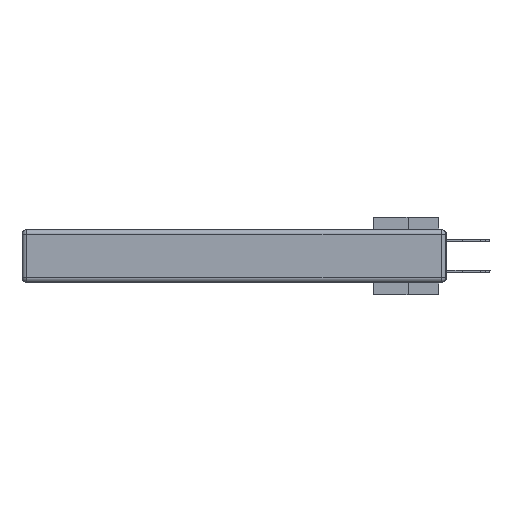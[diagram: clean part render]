
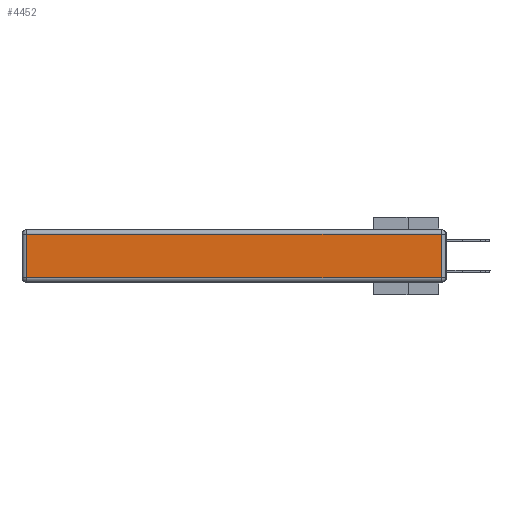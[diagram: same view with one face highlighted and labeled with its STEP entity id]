
A CAD part, left-side view. The second image highlights one B-rep face of the part: STEP entity #4452.
In plain terms, the highlighted planar face has unit normal (-1, 0, 0).
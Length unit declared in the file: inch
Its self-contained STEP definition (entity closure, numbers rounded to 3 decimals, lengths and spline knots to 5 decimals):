
#385 = VERTEX_POINT ( 'NONE', #31252 ) ;
#1004 = EDGE_CURVE ( 'NONE', #385, #21930, #6210, .T. ) ;
#1179 = CARTESIAN_POINT ( 'NONE',  ( 0., 2.72, -0.343 ) ) ;
#1452 = CARTESIAN_POINT ( 'NONE',  ( 0., 0.03, -0.313 ) ) ;
#2350 = EDGE_LOOP ( 'NONE', ( #24834, #15206, #16916, #13776 ) ) ;
#3061 = VECTOR ( 'NONE', #31556, 39.37008 ) ;
#4452 = ADVANCED_FACE ( 'NONE', ( #31015 ), #16796, .T. ) ;
#5399 = EDGE_CURVE ( 'NONE', #21930, #14208, #33611, .T. ) ;
#5431 = DIRECTION ( 'NONE',  ( -1., 0., 0. ) ) ;
#5681 = CARTESIAN_POINT ( 'NONE',  ( 0., 0.03, -0.343 ) ) ;
#6210 = LINE ( 'NONE', #35087, #19211 ) ;
#7542 = LINE ( 'NONE', #1179, #27296 ) ;
#12952 = AXIS2_PLACEMENT_3D ( 'NONE', #22569, #5431, #36917 ) ;
#13776 = ORIENTED_EDGE ( 'NONE', *, *, #34782, .T. ) ;
#14208 = VERTEX_POINT ( 'NONE', #25687 ) ;
#15206 = ORIENTED_EDGE ( 'NONE', *, *, #5399, .T. ) ;
#16582 = DIRECTION ( 'NONE',  ( 0., 0., 1. ) ) ;
#16702 = EDGE_CURVE ( 'NONE', #14208, #31904, #22338, .T. ) ;
#16796 = PLANE ( 'NONE',  #12952 ) ;
#16916 = ORIENTED_EDGE ( 'NONE', *, *, #16702, .T. ) ;
#19211 = VECTOR ( 'NONE', #29871, 39.37008 ) ;
#21930 = VERTEX_POINT ( 'NONE', #1452 ) ;
#22338 = LINE ( 'NONE', #26167, #3061 ) ;
#22569 = CARTESIAN_POINT ( 'NONE',  ( 0., 0., -0.343 ) ) ;
#24834 = ORIENTED_EDGE ( 'NONE', *, *, #1004, .T. ) ;
#25687 = CARTESIAN_POINT ( 'NONE',  ( 0., 0.03, -0.03 ) ) ;
#26167 = CARTESIAN_POINT ( 'NONE',  ( 0., 2.75, -0.03 ) ) ;
#26557 = CARTESIAN_POINT ( 'NONE',  ( 0., 2.72, -0.03 ) ) ;
#27296 = VECTOR ( 'NONE', #33094, 39.37008 ) ;
#27367 = VECTOR ( 'NONE', #16582, 39.37008 ) ;
#29871 = DIRECTION ( 'NONE',  ( 0., -1., 0. ) ) ;
#31015 = FACE_OUTER_BOUND ( 'NONE', #2350, .T. ) ;
#31252 = CARTESIAN_POINT ( 'NONE',  ( 0., 2.72, -0.313 ) ) ;
#31556 = DIRECTION ( 'NONE',  ( 0., 1., 0. ) ) ;
#31904 = VERTEX_POINT ( 'NONE', #26557 ) ;
#33094 = DIRECTION ( 'NONE',  ( 0., 0., -1. ) ) ;
#33611 = LINE ( 'NONE', #5681, #27367 ) ;
#34782 = EDGE_CURVE ( 'NONE', #31904, #385, #7542, .T. ) ;
#35087 = CARTESIAN_POINT ( 'NONE',  ( 0., 0., -0.313 ) ) ;
#36917 = DIRECTION ( 'NONE',  ( 0., 0., 1. ) ) ;
